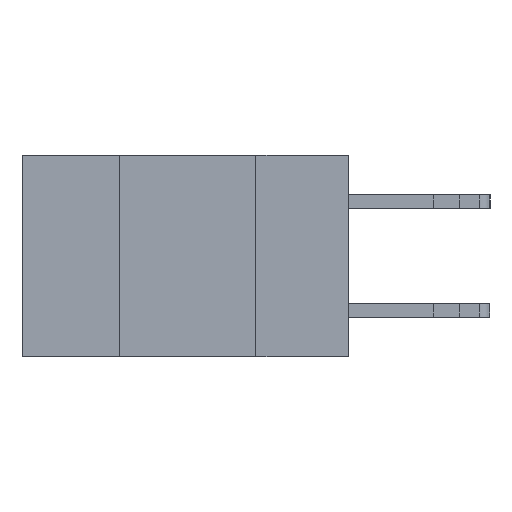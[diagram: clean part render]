
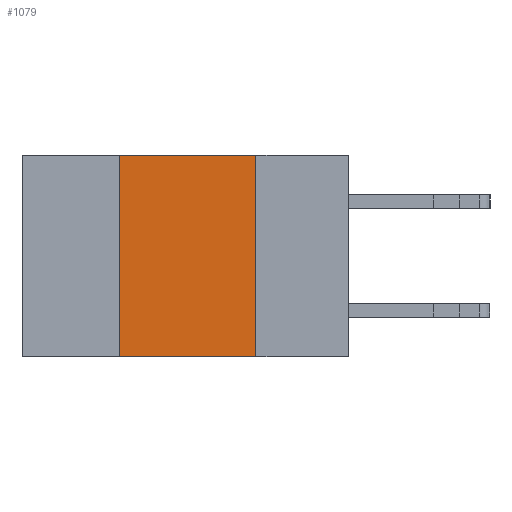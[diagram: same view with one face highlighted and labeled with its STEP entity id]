
A CAD part, left-side view. The second image highlights one B-rep face of the part: STEP entity #1079.
In plain terms, the highlighted planar face has unit normal (-1, 0, 0).
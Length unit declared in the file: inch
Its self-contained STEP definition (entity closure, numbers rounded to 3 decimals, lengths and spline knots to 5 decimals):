
#29 = DIRECTION ( 'NONE',  ( 0., -1., 0. ) ) ;
#358 = EDGE_CURVE ( 'NONE', #5642, #10283, #4889, .T. ) ;
#451 = EDGE_CURVE ( 'NONE', #2794, #10335, #7412, .T. ) ;
#655 = EDGE_CURVE ( 'NONE', #10335, #5642, #4277, .T. ) ;
#786 = PLANE ( 'NONE',  #10921 ) ;
#1079 = ADVANCED_FACE ( 'NONE', ( #4707 ), #786, .F. ) ;
#1279 = LINE ( 'NONE', #4705, #9779 ) ;
#1471 = ORIENTED_EDGE ( 'NONE', *, *, #451, .F. ) ;
#1573 = VECTOR ( 'NONE', #29, 39.37008 ) ;
#2794 = VERTEX_POINT ( 'NONE', #3195 ) ;
#3195 = CARTESIAN_POINT ( 'NONE',  ( 0., 0.42, -0.37 ) ) ;
#3994 = CARTESIAN_POINT ( 'NONE',  ( 0., 0.6, 0. ) ) ;
#4277 = LINE ( 'NONE', #3994, #1573 ) ;
#4705 = CARTESIAN_POINT ( 'NONE',  ( 0., 0.6, -0.37 ) ) ;
#4707 = FACE_OUTER_BOUND ( 'NONE', #7543, .T. ) ;
#4889 = LINE ( 'NONE', #7505, #6822 ) ;
#5054 = ORIENTED_EDGE ( 'NONE', *, *, #10934, .T. ) ;
#5151 = DIRECTION ( 'NONE',  ( 0., 0., 1. ) ) ;
#5258 = CARTESIAN_POINT ( 'NONE',  ( 0., 0.42, 0. ) ) ;
#5642 = VERTEX_POINT ( 'NONE', #6148 ) ;
#6148 = CARTESIAN_POINT ( 'NONE',  ( 0., 0.17, 0. ) ) ;
#6499 = ORIENTED_EDGE ( 'NONE', *, *, #655, .F. ) ;
#6563 = CARTESIAN_POINT ( 'NONE',  ( 0., 0.17, -0.37 ) ) ;
#6777 = CARTESIAN_POINT ( 'NONE',  ( 0., 0.6, 0. ) ) ;
#6822 = VECTOR ( 'NONE', #8214, 39.37008 ) ;
#6857 = ORIENTED_EDGE ( 'NONE', *, *, #358, .F. ) ;
#7040 = VECTOR ( 'NONE', #5151, 39.37008 ) ;
#7412 = LINE ( 'NONE', #5258, #7040 ) ;
#7505 = CARTESIAN_POINT ( 'NONE',  ( 0., 0.17, 0. ) ) ;
#7543 = EDGE_LOOP ( 'NONE', ( #6857, #6499, #1471, #5054 ) ) ;
#7961 = DIRECTION ( 'NONE',  ( 0., -1., 0. ) ) ;
#8214 = DIRECTION ( 'NONE',  ( 0., 0., -1. ) ) ;
#8285 = DIRECTION ( 'NONE',  ( 0., 0., -1. ) ) ;
#9710 = CARTESIAN_POINT ( 'NONE',  ( 0., 0.42, 0. ) ) ;
#9779 = VECTOR ( 'NONE', #7961, 39.37008 ) ;
#10283 = VERTEX_POINT ( 'NONE', #6563 ) ;
#10335 = VERTEX_POINT ( 'NONE', #9710 ) ;
#10828 = DIRECTION ( 'NONE',  ( 1., 0., 0. ) ) ;
#10921 = AXIS2_PLACEMENT_3D ( 'NONE', #6777, #10828, #8285 ) ;
#10934 = EDGE_CURVE ( 'NONE', #2794, #10283, #1279, .T. ) ;
